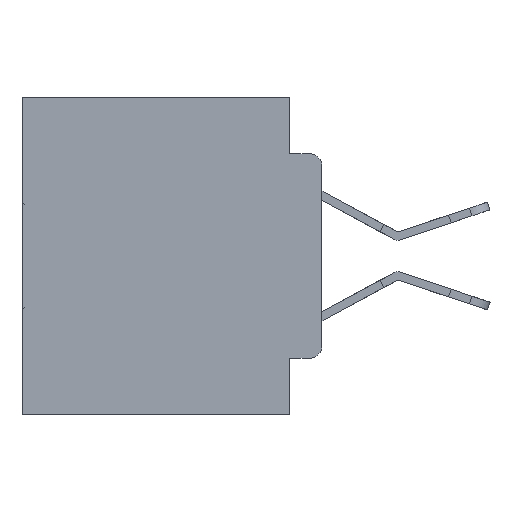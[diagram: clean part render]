
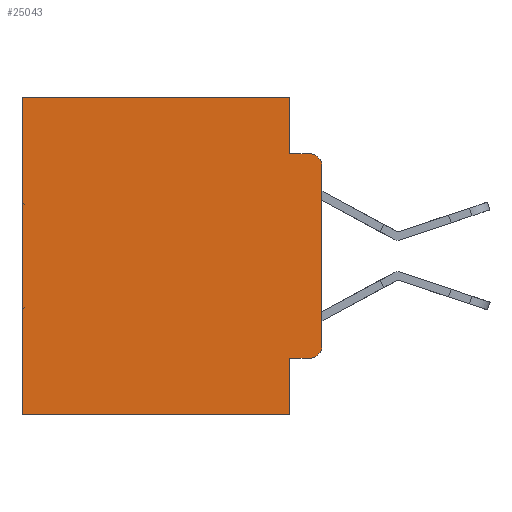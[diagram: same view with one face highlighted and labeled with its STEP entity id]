
A CAD part, left-side view. The second image highlights one B-rep face of the part: STEP entity #25043.
In plain terms, the highlighted planar face has unit normal (-1, 0, 0).
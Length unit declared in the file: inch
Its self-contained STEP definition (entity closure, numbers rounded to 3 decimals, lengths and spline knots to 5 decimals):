
#192 = DIRECTION ( 'NONE',  ( -1., 0., 0. ) ) ;
#221 = CARTESIAN_POINT ( 'NONE',  ( 0.298, 0.473, 0. ) ) ;
#1381 = ORIENTED_EDGE ( 'NONE', *, *, #21769, .F. ) ;
#2455 = CIRCLE ( 'NONE', #19892, 0.02 ) ;
#2585 = ORIENTED_EDGE ( 'NONE', *, *, #12088, .F. ) ;
#2642 = CARTESIAN_POINT ( 'NONE',  ( 0.298, 0.051, -0.4115 ) ) ;
#3017 = DIRECTION ( 'NONE',  ( 0., -1., 0. ) ) ;
#3199 = VERTEX_POINT ( 'NONE', #2642 ) ;
#3299 = VECTOR ( 'NONE', #3721, 39.37008 ) ;
#3721 = DIRECTION ( 'NONE',  ( 0., 0., -1. ) ) ;
#4144 = CARTESIAN_POINT ( 'NONE',  ( 0.298, 0.051, -0.0885 ) ) ;
#4376 = DIRECTION ( 'NONE',  ( 1., 0., 0. ) ) ;
#5759 = ORIENTED_EDGE ( 'NONE', *, *, #9480, .T. ) ;
#6013 = VERTEX_POINT ( 'NONE', #11700 ) ;
#6327 = DIRECTION ( 'NONE',  ( -1., 0., 0. ) ) ;
#6547 = CARTESIAN_POINT ( 'NONE',  ( 0.298, 0.02, -0.1085 ) ) ;
#6739 = EDGE_CURVE ( 'NONE', #28838, #17223, #28266, .T. ) ;
#7298 = VECTOR ( 'NONE', #16168, 39.37008 ) ;
#8804 = AXIS2_PLACEMENT_3D ( 'NONE', #20005, #4376, #25217 ) ;
#8820 = VECTOR ( 'NONE', #25325, 39.37008 ) ;
#9480 = EDGE_CURVE ( 'NONE', #27812, #29936, #28929, .T. ) ;
#9828 = ORIENTED_EDGE ( 'NONE', *, *, #25848, .F. ) ;
#10033 = LINE ( 'NONE', #26583, #21066 ) ;
#10138 = CARTESIAN_POINT ( 'NONE',  ( 0.298, 0.051, 0. ) ) ;
#10316 = CARTESIAN_POINT ( 'NONE',  ( 0.298, 0., -0.5 ) ) ;
#10324 = VERTEX_POINT ( 'NONE', #32448 ) ;
#10487 = AXIS2_PLACEMENT_3D ( 'NONE', #6547, #6327, #11686 ) ;
#10855 = ORIENTED_EDGE ( 'NONE', *, *, #29969, .T. ) ;
#11686 = DIRECTION ( 'NONE',  ( 0., 0., -1. ) ) ;
#11700 = CARTESIAN_POINT ( 'NONE',  ( 0.298, 0.02, -0.4115 ) ) ;
#11900 = PLANE ( 'NONE',  #8804 ) ;
#12088 = EDGE_CURVE ( 'NONE', #3199, #10324, #29843, .T. ) ;
#12605 = LINE ( 'NONE', #10316, #30604 ) ;
#12820 = DIRECTION ( 'NONE',  ( 0., 1., 0. ) ) ;
#13312 = CARTESIAN_POINT ( 'NONE',  ( 0.298, 0.02, -0.3915 ) ) ;
#13333 = LINE ( 'NONE', #4144, #8820 ) ;
#13729 = VERTEX_POINT ( 'NONE', #33279 ) ;
#14714 = EDGE_CURVE ( 'NONE', #3199, #6013, #10033, .T. ) ;
#16168 = DIRECTION ( 'NONE',  ( 0., 1., 0. ) ) ;
#16245 = CARTESIAN_POINT ( 'NONE',  ( 0.298, 0.051, 0. ) ) ;
#17223 = VERTEX_POINT ( 'NONE', #29606 ) ;
#17452 = FACE_OUTER_BOUND ( 'NONE', #29394, .T. ) ;
#17763 = DIRECTION ( 'NONE',  ( 0., 0., -1. ) ) ;
#18189 = VECTOR ( 'NONE', #33752, 39.37008 ) ;
#19262 = LINE ( 'NONE', #221, #20917 ) ;
#19277 = VERTEX_POINT ( 'NONE', #28209 ) ;
#19892 = AXIS2_PLACEMENT_3D ( 'NONE', #13312, #192, #31551 ) ;
#20005 = CARTESIAN_POINT ( 'NONE',  ( 0.298, 0., 0. ) ) ;
#20917 = VECTOR ( 'NONE', #26423, 39.37008 ) ;
#21064 = CARTESIAN_POINT ( 'NONE',  ( 0.298, 0., 0. ) ) ;
#21066 = VECTOR ( 'NONE', #3017, 39.37008 ) ;
#21769 = EDGE_CURVE ( 'NONE', #10324, #23257, #12605, .T. ) ;
#21984 = CARTESIAN_POINT ( 'NONE',  ( 0.298, 0.051, 0. ) ) ;
#22775 = ORIENTED_EDGE ( 'NONE', *, *, #14714, .T. ) ;
#23257 = VERTEX_POINT ( 'NONE', #30617 ) ;
#23369 = VECTOR ( 'NONE', #17763, 39.37008 ) ;
#23900 = CARTESIAN_POINT ( 'NONE',  ( 0.298, 0.473, 0. ) ) ;
#25023 = EDGE_CURVE ( 'NONE', #19277, #13729, #13333, .T. ) ;
#25043 = ADVANCED_FACE ( 'NONE', ( #17452 ), #11900, .F. ) ;
#25217 = DIRECTION ( 'NONE',  ( 0., 0., -1. ) ) ;
#25325 = DIRECTION ( 'NONE',  ( 0., -1., 0. ) ) ;
#25848 = EDGE_CURVE ( 'NONE', #27812, #19277, #33734, .T. ) ;
#26423 = DIRECTION ( 'NONE',  ( 0., 0., -1. ) ) ;
#26583 = CARTESIAN_POINT ( 'NONE',  ( 0.298, 0.051, -0.4115 ) ) ;
#27812 = VERTEX_POINT ( 'NONE', #16245 ) ;
#28209 = CARTESIAN_POINT ( 'NONE',  ( 0.298, 0.051, -0.0885 ) ) ;
#28266 = LINE ( 'NONE', #30414, #23369 ) ;
#28327 = EDGE_CURVE ( 'NONE', #29936, #23257, #19262, .T. ) ;
#28838 = VERTEX_POINT ( 'NONE', #30561 ) ;
#28929 = LINE ( 'NONE', #21064, #7298 ) ;
#29342 = ORIENTED_EDGE ( 'NONE', *, *, #25023, .F. ) ;
#29394 = EDGE_LOOP ( 'NONE', ( #32338, #30818, #29342, #9828, #5759, #30134, #1381, #2585, #22775, #10855 ) ) ;
#29509 = CIRCLE ( 'NONE', #10487, 0.02 ) ;
#29606 = CARTESIAN_POINT ( 'NONE',  ( 0.298, 0., -0.3915 ) ) ;
#29843 = LINE ( 'NONE', #21984, #3299 ) ;
#29936 = VERTEX_POINT ( 'NONE', #23900 ) ;
#29969 = EDGE_CURVE ( 'NONE', #6013, #17223, #2455, .T. ) ;
#30134 = ORIENTED_EDGE ( 'NONE', *, *, #28327, .T. ) ;
#30225 = EDGE_CURVE ( 'NONE', #28838, #13729, #29509, .T. ) ;
#30414 = CARTESIAN_POINT ( 'NONE',  ( 0.298, 0., 0. ) ) ;
#30561 = CARTESIAN_POINT ( 'NONE',  ( 0.298, 0., -0.1085 ) ) ;
#30604 = VECTOR ( 'NONE', #12820, 39.37008 ) ;
#30617 = CARTESIAN_POINT ( 'NONE',  ( 0.298, 0.473, -0.5 ) ) ;
#30818 = ORIENTED_EDGE ( 'NONE', *, *, #30225, .T. ) ;
#31551 = DIRECTION ( 'NONE',  ( 0., 0., -1. ) ) ;
#32338 = ORIENTED_EDGE ( 'NONE', *, *, #6739, .F. ) ;
#32448 = CARTESIAN_POINT ( 'NONE',  ( 0.298, 0.051, -0.5 ) ) ;
#33279 = CARTESIAN_POINT ( 'NONE',  ( 0.298, 0.02, -0.0885 ) ) ;
#33734 = LINE ( 'NONE', #10138, #18189 ) ;
#33752 = DIRECTION ( 'NONE',  ( 0., 0., -1. ) ) ;
